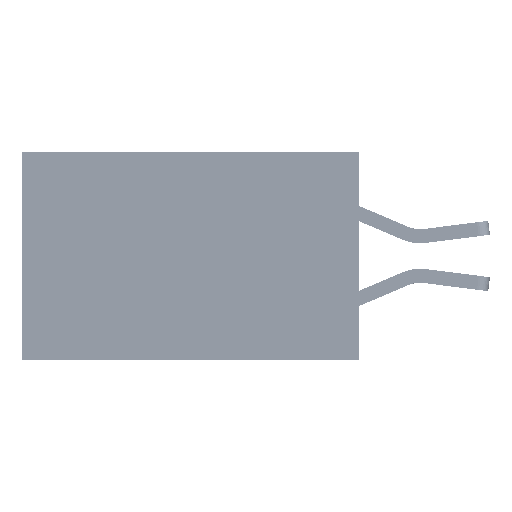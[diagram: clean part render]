
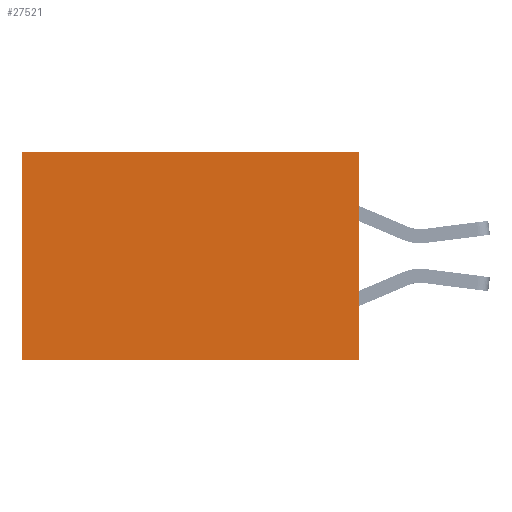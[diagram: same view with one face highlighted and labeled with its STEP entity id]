
A CAD part, left-side view. The second image highlights one B-rep face of the part: STEP entity #27521.
In plain terms, the highlighted planar face has unit normal (-1, 0, 0).
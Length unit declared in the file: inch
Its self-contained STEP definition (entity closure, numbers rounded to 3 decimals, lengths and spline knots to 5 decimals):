
#212 = EDGE_LOOP ( 'NONE', ( #37759, #3879, #9205, #8026 ) ) ;
#264 = CARTESIAN_POINT ( 'NONE',  ( 0.2875, 0., 0. ) ) ;
#1262 = VECTOR ( 'NONE', #19832, 39.37008 ) ;
#1430 = CARTESIAN_POINT ( 'NONE',  ( 0.2875, 0.6, 0. ) ) ;
#1613 = CARTESIAN_POINT ( 'NONE',  ( 0.2875, 0., 0. ) ) ;
#3879 = ORIENTED_EDGE ( 'NONE', *, *, #18806, .F. ) ;
#4968 = VERTEX_POINT ( 'NONE', #35427 ) ;
#6950 = AXIS2_PLACEMENT_3D ( 'NONE', #12408, #12119, #9187 ) ;
#7254 = LINE ( 'NONE', #1613, #11280 ) ;
#8026 = ORIENTED_EDGE ( 'NONE', *, *, #12983, .T. ) ;
#9187 = DIRECTION ( 'NONE',  ( 0., 0., -1. ) ) ;
#9205 = ORIENTED_EDGE ( 'NONE', *, *, #20965, .F. ) ;
#10542 = DIRECTION ( 'NONE',  ( 0., 1., 0. ) ) ;
#10785 = LINE ( 'NONE', #32447, #1262 ) ;
#11280 = VECTOR ( 'NONE', #17020, 39.37008 ) ;
#12119 = DIRECTION ( 'NONE',  ( 1., 0., 0. ) ) ;
#12408 = CARTESIAN_POINT ( 'NONE',  ( 0.2875, 0., 0. ) ) ;
#12983 = EDGE_CURVE ( 'NONE', #23409, #21699, #35505, .T. ) ;
#13486 = CARTESIAN_POINT ( 'NONE',  ( 0.2875, 0., 0. ) ) ;
#14168 = DIRECTION ( 'NONE',  ( 0., 1., 0. ) ) ;
#15925 = FACE_OUTER_BOUND ( 'NONE', #212, .T. ) ;
#17020 = DIRECTION ( 'NONE',  ( 0., 0., -1. ) ) ;
#18806 = EDGE_CURVE ( 'NONE', #4968, #36029, #34508, .T. ) ;
#19832 = DIRECTION ( 'NONE',  ( 0., 0., -1. ) ) ;
#20775 = EDGE_CURVE ( 'NONE', #21699, #36029, #10785, .T. ) ;
#20965 = EDGE_CURVE ( 'NONE', #23409, #4968, #7254, .T. ) ;
#21512 = VECTOR ( 'NONE', #14168, 39.37008 ) ;
#21699 = VERTEX_POINT ( 'NONE', #1430 ) ;
#23409 = VERTEX_POINT ( 'NONE', #264 ) ;
#23526 = VECTOR ( 'NONE', #10542, 39.37008 ) ;
#25166 = PLANE ( 'NONE',  #6950 ) ;
#27521 = ADVANCED_FACE ( 'NONE', ( #15925 ), #25166, .F. ) ;
#32447 = CARTESIAN_POINT ( 'NONE',  ( 0.2875, 0.6, 0. ) ) ;
#34508 = LINE ( 'NONE', #40070, #21512 ) ;
#34736 = CARTESIAN_POINT ( 'NONE',  ( 0.2875, 0.6, -0.37 ) ) ;
#35427 = CARTESIAN_POINT ( 'NONE',  ( 0.2875, 0., -0.37 ) ) ;
#35505 = LINE ( 'NONE', #13486, #23526 ) ;
#36029 = VERTEX_POINT ( 'NONE', #34736 ) ;
#37759 = ORIENTED_EDGE ( 'NONE', *, *, #20775, .T. ) ;
#40070 = CARTESIAN_POINT ( 'NONE',  ( 0.2875, 0., -0.37 ) ) ;
